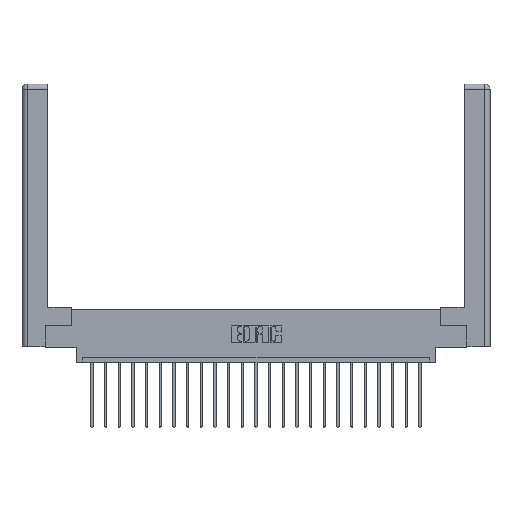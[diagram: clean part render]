
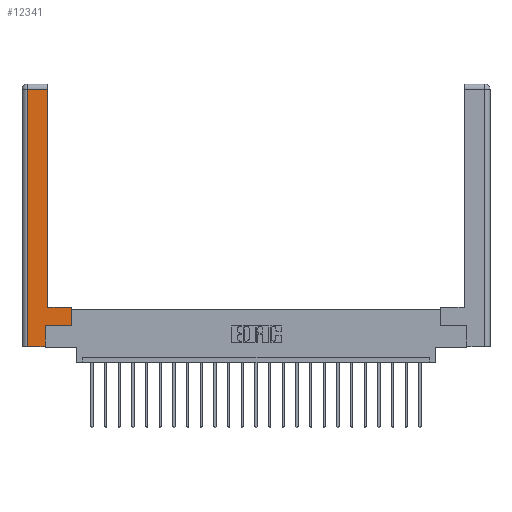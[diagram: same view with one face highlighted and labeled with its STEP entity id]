
A CAD part, top view. The second image highlights one B-rep face of the part: STEP entity #12341.
In plain terms, the highlighted planar face has unit normal (0, 0, 1).
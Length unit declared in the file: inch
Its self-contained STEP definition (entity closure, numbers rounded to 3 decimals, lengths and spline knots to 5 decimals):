
#5 = CARTESIAN_POINT ( 'NONE',  ( 0.0615, 0., 0. ) ) ;
#287 = VECTOR ( 'NONE', #11707, 39.37008 ) ;
#979 = VERTEX_POINT ( 'NONE', #12742 ) ;
#1501 = ORIENTED_EDGE ( 'NONE', *, *, #21204, .T. ) ;
#1648 = VERTEX_POINT ( 'NONE', #23318 ) ;
#2224 = CARTESIAN_POINT ( 'NONE',  ( 0., 0., 0. ) ) ;
#2389 = VERTEX_POINT ( 'NONE', #7933 ) ;
#2413 = DIRECTION ( 'NONE',  ( -1., 0., 0. ) ) ;
#2623 = CARTESIAN_POINT ( 'NONE',  ( 0.0615, 2.94, 0. ) ) ;
#3118 = VERTEX_POINT ( 'NONE', #7848 ) ;
#3775 = EDGE_CURVE ( 'NONE', #16585, #18406, #5277, .T. ) ;
#3945 = ORIENTED_EDGE ( 'NONE', *, *, #17833, .T. ) ;
#3960 = CARTESIAN_POINT ( 'NONE',  ( 0.265, 0., 0. ) ) ;
#4178 = LINE ( 'NONE', #5357, #18167 ) ;
#5230 = DIRECTION ( 'NONE',  ( 0., -1., 0. ) ) ;
#5261 = VECTOR ( 'NONE', #9939, 39.37008 ) ;
#5277 = LINE ( 'NONE', #3960, #13549 ) ;
#5357 = CARTESIAN_POINT ( 'NONE',  ( 0.295, 3., 0. ) ) ;
#5567 = ORIENTED_EDGE ( 'NONE', *, *, #10361, .T. ) ;
#6064 = CARTESIAN_POINT ( 'NONE',  ( 0.0615, 0., 0. ) ) ;
#7848 = CARTESIAN_POINT ( 'NONE',  ( 0.565, 0.245, 0. ) ) ;
#7933 = CARTESIAN_POINT ( 'NONE',  ( 0.295, 0.45, 0. ) ) ;
#8271 = VERTEX_POINT ( 'NONE', #2623 ) ;
#8849 = CARTESIAN_POINT ( 'NONE',  ( 0.565, 0.245, 0. ) ) ;
#8938 = VECTOR ( 'NONE', #21372, 39.37008 ) ;
#9185 = EDGE_CURVE ( 'NONE', #1648, #2389, #12192, .T. ) ;
#9438 = DIRECTION ( 'NONE',  ( 0., 0., -1. ) ) ;
#9554 = AXIS2_PLACEMENT_3D ( 'NONE', #2224, #9438, #18864 ) ;
#9770 = ORIENTED_EDGE ( 'NONE', *, *, #3775, .T. ) ;
#9939 = DIRECTION ( 'NONE',  ( 0., 1., 0. ) ) ;
#10361 = EDGE_CURVE ( 'NONE', #2389, #21560, #4178, .T. ) ;
#10845 = DIRECTION ( 'NONE',  ( 0., 1., 0. ) ) ;
#10943 = DIRECTION ( 'NONE',  ( -1., 0., 0. ) ) ;
#11315 = EDGE_CURVE ( 'NONE', #8271, #16585, #18965, .T. ) ;
#11707 = DIRECTION ( 'NONE',  ( 0., 1., 0. ) ) ;
#11994 = EDGE_CURVE ( 'NONE', #3118, #1648, #14953, .T. ) ;
#12192 = LINE ( 'NONE', #19540, #17952 ) ;
#12341 = ADVANCED_FACE ( 'NONE', ( #21508 ), #13265, .F. ) ;
#12380 = VECTOR ( 'NONE', #5230, 39.37008 ) ;
#12702 = ORIENTED_EDGE ( 'NONE', *, *, #11315, .T. ) ;
#12742 = CARTESIAN_POINT ( 'NONE',  ( 0.265, 0.245, 0. ) ) ;
#13265 = PLANE ( 'NONE',  #9554 ) ;
#13549 = VECTOR ( 'NONE', #21831, 39.37008 ) ;
#14150 = ORIENTED_EDGE ( 'NONE', *, *, #9185, .T. ) ;
#14953 = LINE ( 'NONE', #20806, #5261 ) ;
#15884 = LINE ( 'NONE', #22035, #17044 ) ;
#16016 = CARTESIAN_POINT ( 'NONE',  ( 0.295, 2.94, 0. ) ) ;
#16434 = ORIENTED_EDGE ( 'NONE', *, *, #11994, .T. ) ;
#16460 = EDGE_CURVE ( 'NONE', #21560, #8271, #15884, .T. ) ;
#16585 = VERTEX_POINT ( 'NONE', #6064 ) ;
#16589 = EDGE_LOOP ( 'NONE', ( #5567, #20453, #12702, #9770, #1501, #3945, #16434, #14150 ) ) ;
#17044 = VECTOR ( 'NONE', #10943, 39.37008 ) ;
#17244 = CARTESIAN_POINT ( 'NONE',  ( 0.265, 0.245, 0. ) ) ;
#17833 = EDGE_CURVE ( 'NONE', #979, #3118, #22643, .T. ) ;
#17952 = VECTOR ( 'NONE', #2413, 39.37008 ) ;
#18167 = VECTOR ( 'NONE', #10845, 39.37008 ) ;
#18406 = VERTEX_POINT ( 'NONE', #22859 ) ;
#18782 = LINE ( 'NONE', #17244, #287 ) ;
#18864 = DIRECTION ( 'NONE',  ( -1., 0., 0. ) ) ;
#18965 = LINE ( 'NONE', #5, #12380 ) ;
#19540 = CARTESIAN_POINT ( 'NONE',  ( 0.295, 0.45, 0. ) ) ;
#20453 = ORIENTED_EDGE ( 'NONE', *, *, #16460, .T. ) ;
#20806 = CARTESIAN_POINT ( 'NONE',  ( 0.565, 0.45, 0. ) ) ;
#21204 = EDGE_CURVE ( 'NONE', #18406, #979, #18782, .T. ) ;
#21372 = DIRECTION ( 'NONE',  ( 1., 0., 0. ) ) ;
#21508 = FACE_OUTER_BOUND ( 'NONE', #16589, .T. ) ;
#21560 = VERTEX_POINT ( 'NONE', #16016 ) ;
#21831 = DIRECTION ( 'NONE',  ( 1., 0., 0. ) ) ;
#22035 = CARTESIAN_POINT ( 'NONE',  ( 0.0615, 2.94, 0. ) ) ;
#22643 = LINE ( 'NONE', #8849, #8938 ) ;
#22859 = CARTESIAN_POINT ( 'NONE',  ( 0.265, 0., 0. ) ) ;
#23318 = CARTESIAN_POINT ( 'NONE',  ( 0.565, 0.45, 0. ) ) ;
